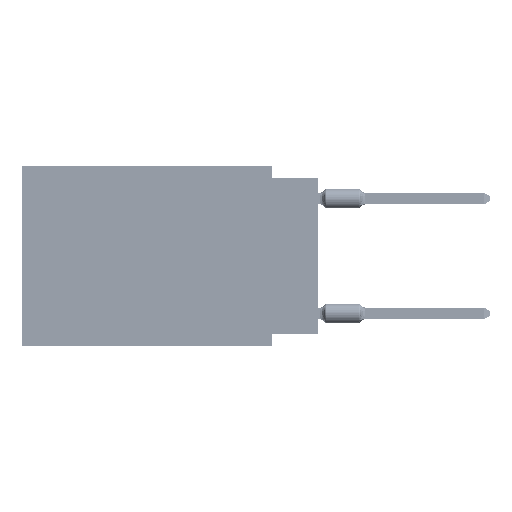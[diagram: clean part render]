
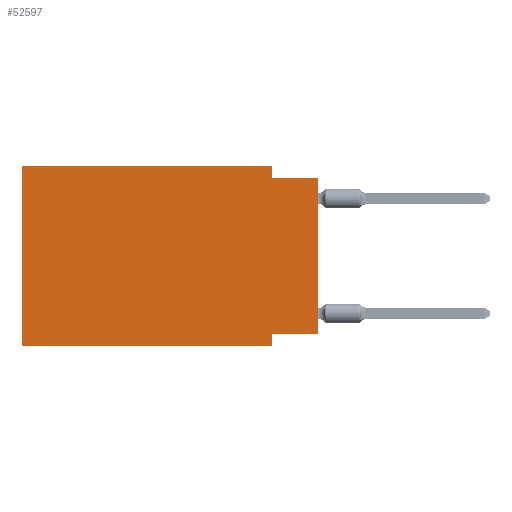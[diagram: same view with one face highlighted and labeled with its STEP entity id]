
A CAD part, left-side view. The second image highlights one B-rep face of the part: STEP entity #52597.
In plain terms, the highlighted planar face has unit normal (-1, 0, 0).
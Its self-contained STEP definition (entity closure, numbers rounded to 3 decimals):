
#97 = CARTESIAN_POINT ( 'NONE',  ( 0., 16.383, 0. ) ) ;
#929 = DIRECTION ( 'NONE',  ( 0., -1., 0. ) ) ;
#1349 = ORIENTED_EDGE ( 'NONE', *, *, #9657, .T. ) ;
#1983 = ORIENTED_EDGE ( 'NONE', *, *, #41053, .T. ) ;
#2216 = CARTESIAN_POINT ( 'NONE',  ( 0., 2.54, -0.635 ) ) ;
#4526 = LINE ( 'NONE', #54088, #27360 ) ;
#5331 = DIRECTION ( 'NONE',  ( 0., 0., -1. ) ) ;
#6204 = ORIENTED_EDGE ( 'NONE', *, *, #18509, .F. ) ;
#7426 = CARTESIAN_POINT ( 'NONE',  ( 0., 16.383, -9.906 ) ) ;
#8176 = ORIENTED_EDGE ( 'NONE', *, *, #24128, .F. ) ;
#9346 = LINE ( 'NONE', #41036, #39767 ) ;
#9657 = EDGE_CURVE ( 'NONE', #56644, #33833, #76427, .T. ) ;
#10352 = LINE ( 'NONE', #21724, #22146 ) ;
#10883 = VERTEX_POINT ( 'NONE', #12442 ) ;
#11494 = LINE ( 'NONE', #97, #16541 ) ;
#12234 = FACE_OUTER_BOUND ( 'NONE', #62005, .T. ) ;
#12442 = CARTESIAN_POINT ( 'NONE',  ( 0., 2.54, 0. ) ) ;
#13367 = ORIENTED_EDGE ( 'NONE', *, *, #63302, .F. ) ;
#14383 = CARTESIAN_POINT ( 'NONE',  ( 0., 16.383, 0. ) ) ;
#14438 = DIRECTION ( 'NONE',  ( 0., 0., 1. ) ) ;
#15768 = VERTEX_POINT ( 'NONE', #26422 ) ;
#16182 = CARTESIAN_POINT ( 'NONE',  ( 0., 16.383, -9.906 ) ) ;
#16541 = VECTOR ( 'NONE', #61844, 1000. ) ;
#17908 = CARTESIAN_POINT ( 'NONE',  ( 0., 16.383, 0. ) ) ;
#18509 = EDGE_CURVE ( 'NONE', #56644, #55563, #47177, .T. ) ;
#19425 = VECTOR ( 'NONE', #28508, 1000. ) ;
#21323 = DIRECTION ( 'NONE',  ( 0., -1., 0. ) ) ;
#21724 = CARTESIAN_POINT ( 'NONE',  ( 0., 0., -0.635 ) ) ;
#22146 = VECTOR ( 'NONE', #21323, 1000. ) ;
#22407 = DIRECTION ( 'NONE',  ( 0., 0., -1. ) ) ;
#23667 = VERTEX_POINT ( 'NONE', #64780 ) ;
#24013 = CARTESIAN_POINT ( 'NONE',  ( 0., 16.383, 0. ) ) ;
#24128 = EDGE_CURVE ( 'NONE', #10883, #49968, #40718, .T. ) ;
#26422 = CARTESIAN_POINT ( 'NONE',  ( 0., 0., -9.271 ) ) ;
#27264 = ORIENTED_EDGE ( 'NONE', *, *, #48223, .F. ) ;
#27360 = VECTOR ( 'NONE', #22407, 1000. ) ;
#28508 = DIRECTION ( 'NONE',  ( 0., 0., 1. ) ) ;
#33018 = CARTESIAN_POINT ( 'NONE',  ( 0., 2.54, 0. ) ) ;
#33833 = VERTEX_POINT ( 'NONE', #77001 ) ;
#39619 = LINE ( 'NONE', #46120, #51251 ) ;
#39767 = VECTOR ( 'NONE', #77136, 1000. ) ;
#40718 = LINE ( 'NONE', #33018, #62090 ) ;
#41036 = CARTESIAN_POINT ( 'NONE',  ( 0., 0., -9.271 ) ) ;
#41053 = EDGE_CURVE ( 'NONE', #15768, #23667, #39619, .T. ) ;
#41898 = CARTESIAN_POINT ( 'NONE',  ( 0., 2.54, -9.271 ) ) ;
#43931 = EDGE_CURVE ( 'NONE', #15768, #64519, #9346, .T. ) ;
#46120 = CARTESIAN_POINT ( 'NONE',  ( 0., 0., 0. ) ) ;
#47177 = LINE ( 'NONE', #24013, #19425 ) ;
#48223 = EDGE_CURVE ( 'NONE', #49968, #23667, #10352, .T. ) ;
#48791 = PLANE ( 'NONE',  #79361 ) ;
#49968 = VERTEX_POINT ( 'NONE', #2216 ) ;
#51251 = VECTOR ( 'NONE', #14438, 1000. ) ;
#52597 = ADVANCED_FACE ( 'NONE', ( #12234 ), #48791, .F. ) ;
#54088 = CARTESIAN_POINT ( 'NONE',  ( 0., 2.54, -9.906 ) ) ;
#55563 = VERTEX_POINT ( 'NONE', #14383 ) ;
#56644 = VERTEX_POINT ( 'NONE', #16182 ) ;
#58985 = DIRECTION ( 'NONE',  ( 0., 0., -1. ) ) ;
#60979 = DIRECTION ( 'NONE',  ( 1., 0., 0. ) ) ;
#61844 = DIRECTION ( 'NONE',  ( 0., -1., 0. ) ) ;
#62005 = EDGE_LOOP ( 'NONE', ( #1983, #27264, #8176, #62297, #6204, #1349, #13367, #66254 ) ) ;
#62090 = VECTOR ( 'NONE', #58985, 1000. ) ;
#62297 = ORIENTED_EDGE ( 'NONE', *, *, #68421, .F. ) ;
#63302 = EDGE_CURVE ( 'NONE', #64519, #33833, #4526, .T. ) ;
#64519 = VERTEX_POINT ( 'NONE', #41898 ) ;
#64780 = CARTESIAN_POINT ( 'NONE',  ( 0., 0., -0.635 ) ) ;
#66254 = ORIENTED_EDGE ( 'NONE', *, *, #43931, .F. ) ;
#68421 = EDGE_CURVE ( 'NONE', #55563, #10883, #11494, .T. ) ;
#76427 = LINE ( 'NONE', #7426, #76901 ) ;
#76901 = VECTOR ( 'NONE', #929, 1000. ) ;
#77001 = CARTESIAN_POINT ( 'NONE',  ( 0., 2.54, -9.906 ) ) ;
#77136 = DIRECTION ( 'NONE',  ( 0., 1., 0. ) ) ;
#79361 = AXIS2_PLACEMENT_3D ( 'NONE', #17908, #60979, #5331 ) ;
